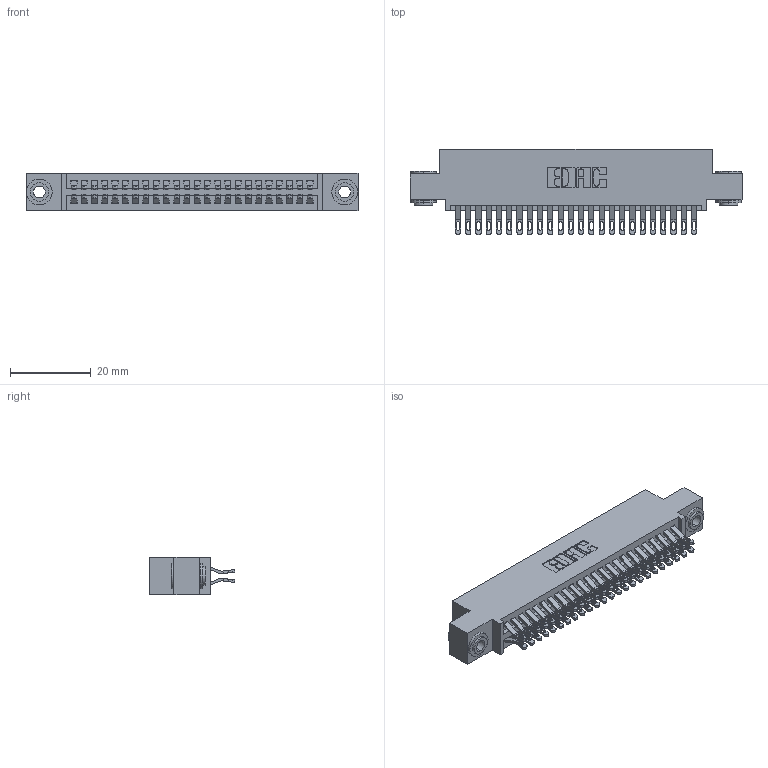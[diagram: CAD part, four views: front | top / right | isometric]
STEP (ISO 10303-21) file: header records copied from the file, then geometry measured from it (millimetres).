
FILE_DESCRIPTION (( 'STEP AP203' ), '1' );
FILE_NAME ('395-048-555-503.STEP', '2018-11-19T22:19:13', ( '' ), ( '' ), 'SwSTEP 2.0', 'SolidWorks 2016', '' );
FILE_SCHEMA (( 'CONFIG_CONTROL_DESIGN' ));
Length unit declared in the file: inch
Products named in the file (4): 345 Part_0.110 Offset - 0.156 Dia-TH; 345-292-001_555 Tail; 345-250-002_345-250-002-102; 395-048-555-503
Assembly tree (51 placements, depth 2):
  395-048-555-503
    345 Part_0.110 Offset - 0.156 Dia-TH
    345-292-001_555 Tail  x48
    345-250-002_345-250-002-102  x2
Bounding box: 82.17 x 21.13 x 9.4 mm (x, y, z)
Volume: 7900.2 mm3; surface area: 12111.1 mm2
Topology: 51 solids, 51 shells, 2856 faces, 8925 edges, 5946 vertices
Faces by surface type: plane 1582, cylinder 1266, cone 8
Entity records: 22362 total; most frequent: CARTESIAN_POINT 3777, ORIENTED_EDGE 3674, DIRECTION 3351, EDGE_CURVE 1837, LINE 1565, VECTOR 1565, VERTEX_POINT 1222, AXIS2_PLACEMENT_3D 893
